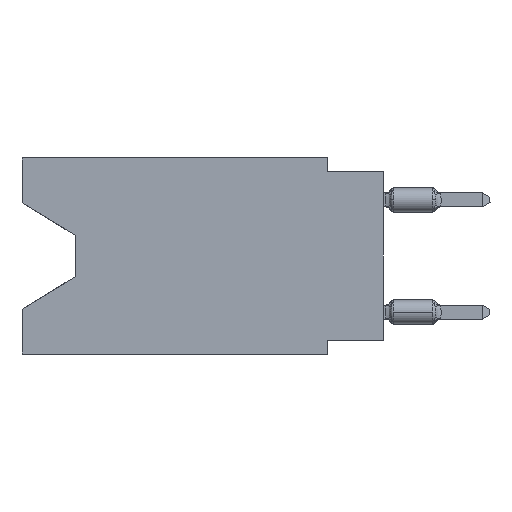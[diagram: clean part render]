
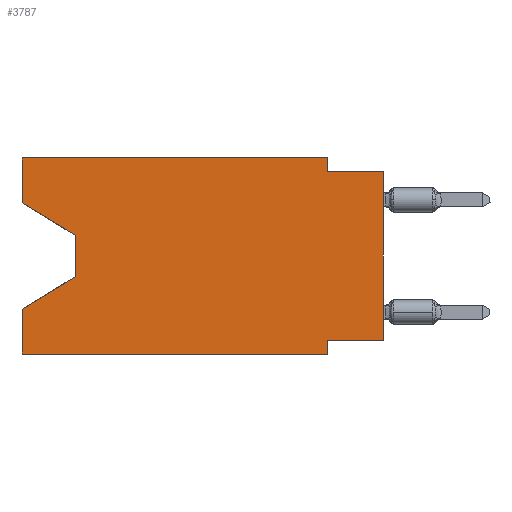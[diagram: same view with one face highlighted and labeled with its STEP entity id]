
A CAD part, left-side view. The second image highlights one B-rep face of the part: STEP entity #3787.
In plain terms, the highlighted planar face has unit normal (-1, 0, 0).
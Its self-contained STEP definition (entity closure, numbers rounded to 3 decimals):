
#534 = LINE ( 'NONE', #15921, #5531 ) ;
#609 = CARTESIAN_POINT ( 'NONE',  ( 0., 0., -0.635 ) ) ;
#820 = DIRECTION ( 'NONE',  ( 0., -1., 0. ) ) ;
#828 = VERTEX_POINT ( 'NONE', #14047 ) ;
#867 = DIRECTION ( 'NONE',  ( 0., 0., -1. ) ) ;
#975 = ORIENTED_EDGE ( 'NONE', *, *, #12371, .F. ) ;
#1021 = EDGE_CURVE ( 'NONE', #11681, #4564, #13520, .T. ) ;
#1261 = LINE ( 'NONE', #20029, #10143 ) ;
#2058 = VECTOR ( 'NONE', #5581, 1000. ) ;
#2308 = CARTESIAN_POINT ( 'NONE',  ( 0., 2.54, -8.89 ) ) ;
#2559 = VECTOR ( 'NONE', #16746, 1000. ) ;
#2636 = CARTESIAN_POINT ( 'NONE',  ( 0., 2.54, -0.635 ) ) ;
#2713 = LINE ( 'NONE', #18204, #16176 ) ;
#2740 = ORIENTED_EDGE ( 'NONE', *, *, #1021, .F. ) ;
#2996 = VERTEX_POINT ( 'NONE', #2636 ) ;
#3321 = LINE ( 'NONE', #18820, #10390 ) ;
#3500 = VECTOR ( 'NONE', #867, 1000. ) ;
#3787 = ADVANCED_FACE ( 'NONE', ( #7071 ), #12008, .F. ) ;
#3965 = DIRECTION ( 'NONE',  ( 0., 0., 1. ) ) ;
#4359 = EDGE_CURVE ( 'NONE', #15750, #828, #11628, .T. ) ;
#4564 = VERTEX_POINT ( 'NONE', #13689 ) ;
#4704 = VECTOR ( 'NONE', #16802, 1000. ) ;
#5358 = CARTESIAN_POINT ( 'NONE',  ( 0., 13.97, -3.505 ) ) ;
#5531 = VECTOR ( 'NONE', #8213, 1000. ) ;
#5581 = DIRECTION ( 'NONE',  ( 0., 1., 0. ) ) ;
#5672 = VERTEX_POINT ( 'NONE', #14159 ) ;
#6094 = AXIS2_PLACEMENT_3D ( 'NONE', #8928, #15197, #7382 ) ;
#6198 = EDGE_CURVE ( 'NONE', #11914, #17115, #10503, .T. ) ;
#6974 = CARTESIAN_POINT ( 'NONE',  ( 0., 0., 0. ) ) ;
#7071 = FACE_OUTER_BOUND ( 'NONE', #19674, .T. ) ;
#7219 = ORIENTED_EDGE ( 'NONE', *, *, #10293, .T. ) ;
#7382 = DIRECTION ( 'NONE',  ( 0., 0., -1. ) ) ;
#7414 = EDGE_CURVE ( 'NONE', #2996, #5672, #14650, .T. ) ;
#7809 = CARTESIAN_POINT ( 'NONE',  ( 0., 16.383, -8.89 ) ) ;
#8213 = DIRECTION ( 'NONE',  ( 0., 0., -1. ) ) ;
#8646 = ORIENTED_EDGE ( 'NONE', *, *, #8667, .T. ) ;
#8667 = EDGE_CURVE ( 'NONE', #17553, #15750, #14657, .T. ) ;
#8799 = LINE ( 'NONE', #15057, #20217 ) ;
#8928 = CARTESIAN_POINT ( 'NONE',  ( 0., 16.383, 0. ) ) ;
#8932 = VERTEX_POINT ( 'NONE', #9808 ) ;
#9672 = VECTOR ( 'NONE', #3965, 1000. ) ;
#9808 = CARTESIAN_POINT ( 'NONE',  ( 0., 2.54, 0. ) ) ;
#10024 = CARTESIAN_POINT ( 'NONE',  ( 0., 16.383, -2.038 ) ) ;
#10072 = ORIENTED_EDGE ( 'NONE', *, *, #7414, .F. ) ;
#10143 = VECTOR ( 'NONE', #19721, 1000. ) ;
#10293 = EDGE_CURVE ( 'NONE', #11914, #5672, #19930, .T. ) ;
#10390 = VECTOR ( 'NONE', #20164, 1000. ) ;
#10449 = LINE ( 'NONE', #19700, #15884 ) ;
#10500 = DIRECTION ( 'NONE',  ( 0., 0., -1. ) ) ;
#10503 = LINE ( 'NONE', #19657, #2058 ) ;
#11628 = LINE ( 'NONE', #5358, #3500 ) ;
#11681 = VERTEX_POINT ( 'NONE', #7809 ) ;
#11914 = VERTEX_POINT ( 'NONE', #14975 ) ;
#12008 = PLANE ( 'NONE',  #6094 ) ;
#12218 = CARTESIAN_POINT ( 'NONE',  ( 0., 16.383, -2.038 ) ) ;
#12371 = EDGE_CURVE ( 'NONE', #17601, #8932, #8799, .T. ) ;
#13520 = LINE ( 'NONE', #14951, #9672 ) ;
#13689 = CARTESIAN_POINT ( 'NONE',  ( 0., 16.383, -6.852 ) ) ;
#14047 = CARTESIAN_POINT ( 'NONE',  ( 0., 13.97, -5.385 ) ) ;
#14159 = CARTESIAN_POINT ( 'NONE',  ( 0., 0., -0.635 ) ) ;
#14458 = ORIENTED_EDGE ( 'NONE', *, *, #18162, .F. ) ;
#14525 = ORIENTED_EDGE ( 'NONE', *, *, #17454, .T. ) ;
#14650 = LINE ( 'NONE', #609, #4704 ) ;
#14657 = LINE ( 'NONE', #10024, #16449 ) ;
#14819 = EDGE_CURVE ( 'NONE', #17553, #17601, #3321, .T. ) ;
#14951 = CARTESIAN_POINT ( 'NONE',  ( 0., 16.383, 0. ) ) ;
#14956 = DIRECTION ( 'NONE',  ( 0., -0.855, -0.519 ) ) ;
#14975 = CARTESIAN_POINT ( 'NONE',  ( 0., 0., -8.255 ) ) ;
#15057 = CARTESIAN_POINT ( 'NONE',  ( 0., 16.383, 0. ) ) ;
#15197 = DIRECTION ( 'NONE',  ( 1., 0., 0. ) ) ;
#15750 = VERTEX_POINT ( 'NONE', #20018 ) ;
#15884 = VECTOR ( 'NONE', #820, 1000. ) ;
#15921 = CARTESIAN_POINT ( 'NONE',  ( 0., 2.54, -8.89 ) ) ;
#16176 = VECTOR ( 'NONE', #10500, 1000. ) ;
#16270 = VERTEX_POINT ( 'NONE', #2308 ) ;
#16449 = VECTOR ( 'NONE', #14956, 1000. ) ;
#16494 = CARTESIAN_POINT ( 'NONE',  ( 0., 2.54, -8.255 ) ) ;
#16746 = DIRECTION ( 'NONE',  ( 0., 0., 1. ) ) ;
#16756 = EDGE_CURVE ( 'NONE', #17115, #16270, #534, .T. ) ;
#16781 = ORIENTED_EDGE ( 'NONE', *, *, #4359, .T. ) ;
#16802 = DIRECTION ( 'NONE',  ( 0., -1., 0. ) ) ;
#17053 = CARTESIAN_POINT ( 'NONE',  ( 0., 16.383, 0. ) ) ;
#17115 = VERTEX_POINT ( 'NONE', #16494 ) ;
#17325 = ORIENTED_EDGE ( 'NONE', *, *, #19020, .T. ) ;
#17454 = EDGE_CURVE ( 'NONE', #828, #4564, #1261, .T. ) ;
#17553 = VERTEX_POINT ( 'NONE', #12218 ) ;
#17601 = VERTEX_POINT ( 'NONE', #17053 ) ;
#18162 = EDGE_CURVE ( 'NONE', #8932, #2996, #2713, .T. ) ;
#18204 = CARTESIAN_POINT ( 'NONE',  ( 0., 2.54, 0. ) ) ;
#18461 = ORIENTED_EDGE ( 'NONE', *, *, #16756, .F. ) ;
#18820 = CARTESIAN_POINT ( 'NONE',  ( 0., 16.383, 0. ) ) ;
#19020 = EDGE_CURVE ( 'NONE', #11681, #16270, #10449, .T. ) ;
#19367 = DIRECTION ( 'NONE',  ( 0., -1., 0. ) ) ;
#19657 = CARTESIAN_POINT ( 'NONE',  ( 0., 0., -8.255 ) ) ;
#19674 = EDGE_LOOP ( 'NONE', ( #8646, #16781, #14525, #2740, #17325, #18461, #19950, #7219, #10072, #14458, #975, #20118 ) ) ;
#19700 = CARTESIAN_POINT ( 'NONE',  ( 0., 16.383, -8.89 ) ) ;
#19721 = DIRECTION ( 'NONE',  ( 0., 0.855, -0.519 ) ) ;
#19930 = LINE ( 'NONE', #6974, #2559 ) ;
#19950 = ORIENTED_EDGE ( 'NONE', *, *, #6198, .F. ) ;
#20018 = CARTESIAN_POINT ( 'NONE',  ( 0., 13.97, -3.505 ) ) ;
#20029 = CARTESIAN_POINT ( 'NONE',  ( 0., 13.97, -5.385 ) ) ;
#20118 = ORIENTED_EDGE ( 'NONE', *, *, #14819, .F. ) ;
#20164 = DIRECTION ( 'NONE',  ( 0., 0., 1. ) ) ;
#20217 = VECTOR ( 'NONE', #19367, 1000. ) ;
